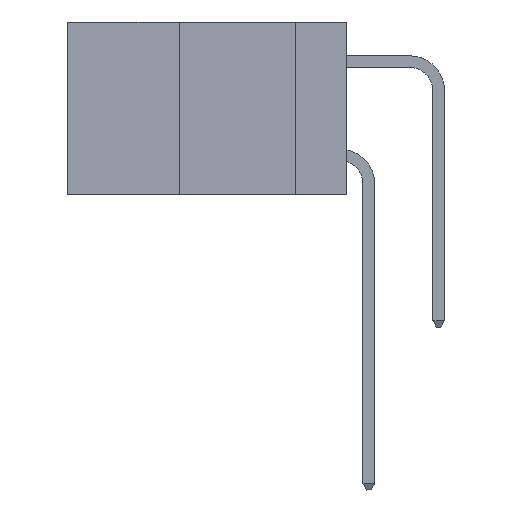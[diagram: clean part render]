
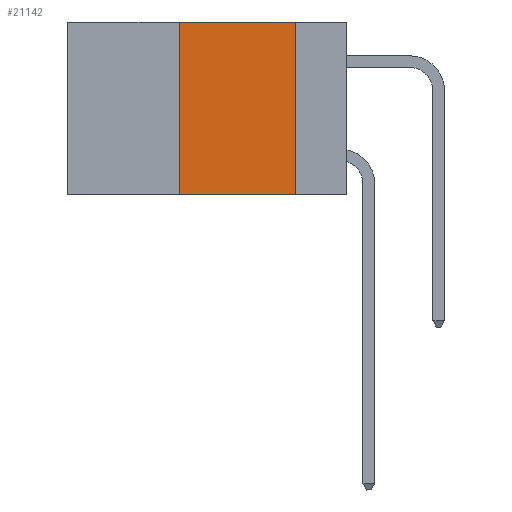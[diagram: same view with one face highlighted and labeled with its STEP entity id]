
A CAD part, left-side view. The second image highlights one B-rep face of the part: STEP entity #21142.
In plain terms, the highlighted planar face has unit normal (-1, 0, 0).
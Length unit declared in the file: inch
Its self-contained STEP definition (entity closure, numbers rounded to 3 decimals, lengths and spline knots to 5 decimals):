
#1401 = DIRECTION ( 'NONE',  ( 0., 0., -1. ) ) ;
#1551 = VECTOR ( 'NONE', #23607, 39.37008 ) ;
#2039 = CARTESIAN_POINT ( 'NONE',  ( 0., 0.11, 0. ) ) ;
#2180 = VERTEX_POINT ( 'NONE', #4912 ) ;
#2342 = CARTESIAN_POINT ( 'NONE',  ( 0., 0.36, 0. ) ) ;
#2457 = AXIS2_PLACEMENT_3D ( 'NONE', #22656, #24851, #1401 ) ;
#2553 = EDGE_CURVE ( 'NONE', #2180, #3136, #23930, .T. ) ;
#3136 = VERTEX_POINT ( 'NONE', #10653 ) ;
#3258 = VECTOR ( 'NONE', #29167, 39.37008 ) ;
#3677 = LINE ( 'NONE', #22470, #6498 ) ;
#4480 = VECTOR ( 'NONE', #14935, 39.37008 ) ;
#4912 = CARTESIAN_POINT ( 'NONE',  ( 0., 0.36, -0.37 ) ) ;
#6161 = ORIENTED_EDGE ( 'NONE', *, *, #25702, .F. ) ;
#6498 = VECTOR ( 'NONE', #8026, 39.37008 ) ;
#8026 = DIRECTION ( 'NONE',  ( 0., 0., 1. ) ) ;
#8261 = VERTEX_POINT ( 'NONE', #2342 ) ;
#10653 = CARTESIAN_POINT ( 'NONE',  ( 0., 0.11, -0.37 ) ) ;
#11016 = FACE_OUTER_BOUND ( 'NONE', #17277, .T. ) ;
#12113 = LINE ( 'NONE', #21580, #3258 ) ;
#14935 = DIRECTION ( 'NONE',  ( 0., 0., -1. ) ) ;
#15023 = EDGE_CURVE ( 'NONE', #8261, #19602, #12113, .T. ) ;
#17277 = EDGE_LOOP ( 'NONE', ( #20697, #27124, #6161, #25246 ) ) ;
#17403 = LINE ( 'NONE', #22203, #4480 ) ;
#19602 = VERTEX_POINT ( 'NONE', #2039 ) ;
#20697 = ORIENTED_EDGE ( 'NONE', *, *, #28013, .F. ) ;
#21142 = ADVANCED_FACE ( 'NONE', ( #11016 ), #23110, .F. ) ;
#21580 = CARTESIAN_POINT ( 'NONE',  ( 0., 0.6, 0. ) ) ;
#22203 = CARTESIAN_POINT ( 'NONE',  ( 0., 0.11, 0. ) ) ;
#22470 = CARTESIAN_POINT ( 'NONE',  ( 0., 0.36, 0. ) ) ;
#22656 = CARTESIAN_POINT ( 'NONE',  ( 0., 0.6, 0. ) ) ;
#23110 = PLANE ( 'NONE',  #2457 ) ;
#23607 = DIRECTION ( 'NONE',  ( 0., -1., 0. ) ) ;
#23930 = LINE ( 'NONE', #28247, #1551 ) ;
#24851 = DIRECTION ( 'NONE',  ( 1., 0., 0. ) ) ;
#25246 = ORIENTED_EDGE ( 'NONE', *, *, #2553, .T. ) ;
#25702 = EDGE_CURVE ( 'NONE', #2180, #8261, #3677, .T. ) ;
#27124 = ORIENTED_EDGE ( 'NONE', *, *, #15023, .F. ) ;
#28013 = EDGE_CURVE ( 'NONE', #19602, #3136, #17403, .T. ) ;
#28247 = CARTESIAN_POINT ( 'NONE',  ( 0., 0.6, -0.37 ) ) ;
#29167 = DIRECTION ( 'NONE',  ( 0., -1., 0. ) ) ;
